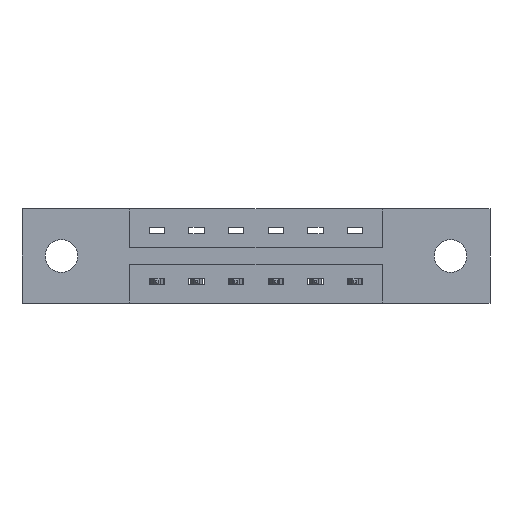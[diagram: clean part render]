
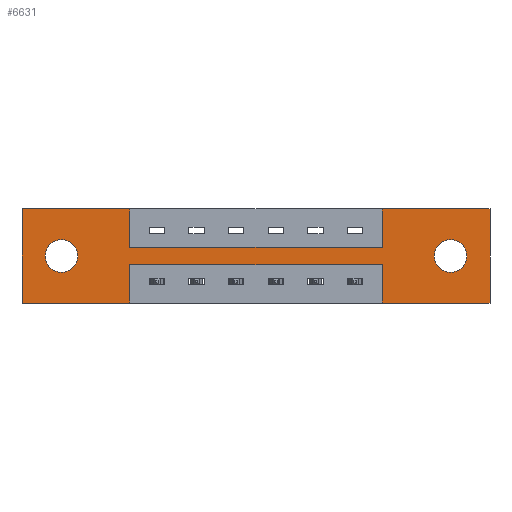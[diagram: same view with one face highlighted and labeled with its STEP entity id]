
A CAD part, front view. The second image highlights one B-rep face of the part: STEP entity #6631.
In plain terms, the highlighted planar face has unit normal (0, -1, 0).
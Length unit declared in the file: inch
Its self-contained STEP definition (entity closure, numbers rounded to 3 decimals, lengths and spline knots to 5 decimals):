
#16 = VERTEX_POINT ( 'NONE', #6132 ) ;
#101 = EDGE_LOOP ( 'NONE', ( #5256, #5325, #5389, #5403, #5441, #5453, #5477, #5502, #5543, #5580, #5597, #5687 ) ) ;
#127 = CIRCLE ( 'NONE', #4814, 0.064 ) ;
#151 = CARTESIAN_POINT ( 'NONE',  ( 1.417, 0., -0.15 ) ) ;
#160 = CARTESIAN_POINT ( 'NONE',  ( 0., 0., 0. ) ) ;
#182 = EDGE_CURVE ( 'NONE', #6004, #833, #659, .T. ) ;
#189 = CIRCLE ( 'NONE', #5176, 0.064 ) ;
#208 = DIRECTION ( 'NONE',  ( 0., 0., -1. ) ) ;
#209 = AXIS2_PLACEMENT_3D ( 'NONE', #7320, #3175, #2017 ) ;
#292 = CARTESIAN_POINT ( 'NONE',  ( 1.842, 0., -0.37 ) ) ;
#468 = DIRECTION ( 'NONE',  ( 1., 0., 0. ) ) ;
#531 = EDGE_CURVE ( 'NONE', #5519, #2962, #932, .T. ) ;
#544 = DIRECTION ( 'NONE',  ( -1., 0., 0. ) ) ;
#653 = CARTESIAN_POINT ( 'NONE',  ( 0.425, 0., 0. ) ) ;
#659 = LINE ( 'NONE', #3459, #2836 ) ;
#678 = VECTOR ( 'NONE', #828, 39.37008 ) ;
#758 = VECTOR ( 'NONE', #3365, 39.37008 ) ;
#828 = DIRECTION ( 'NONE',  ( -1., 0., 0. ) ) ;
#833 = VERTEX_POINT ( 'NONE', #1382 ) ;
#862 = EDGE_CURVE ( 'NONE', #2962, #3034, #5804, .T. ) ;
#932 = LINE ( 'NONE', #8737, #3050 ) ;
#995 = FACE_BOUND ( 'NONE', #5242, .T. ) ;
#1085 = EDGE_CURVE ( 'NONE', #6844, #3231, #1490, .T. ) ;
#1137 = DIRECTION ( 'NONE',  ( 0., 0., 1. ) ) ;
#1150 = CARTESIAN_POINT ( 'NONE',  ( 1.417, 0., 0. ) ) ;
#1175 = EDGE_CURVE ( 'NONE', #7182, #4051, #189, .T. ) ;
#1299 = EDGE_CURVE ( 'NONE', #16, #2086, #6705, .T. ) ;
#1382 = CARTESIAN_POINT ( 'NONE',  ( 0.425, 0., -0.15 ) ) ;
#1426 = VECTOR ( 'NONE', #468, 39.37008 ) ;
#1449 = CARTESIAN_POINT ( 'NONE',  ( 0.155, 0., -0.185 ) ) ;
#1450 = CARTESIAN_POINT ( 'NONE',  ( 0., 0., 0. ) ) ;
#1486 = EDGE_LOOP ( 'NONE', ( #5224, #5228 ) ) ;
#1490 = CIRCLE ( 'NONE', #1927, 0.064 ) ;
#1765 = EDGE_CURVE ( 'NONE', #3231, #6844, #127, .T. ) ;
#1921 = VECTOR ( 'NONE', #3232, 39.37008 ) ;
#1927 = AXIS2_PLACEMENT_3D ( 'NONE', #9051, #9048, #8872 ) ;
#1930 = DIRECTION ( 'NONE',  ( 0., 1., 0. ) ) ;
#1957 = EDGE_CURVE ( 'NONE', #4051, #7182, #5655, .T. ) ;
#1971 = EDGE_CURVE ( 'NONE', #8786, #16, #8321, .T. ) ;
#1974 = EDGE_CURVE ( 'NONE', #2156, #8786, #5214, .T. ) ;
#2004 = EDGE_CURVE ( 'NONE', #5467, #6004, #8154, .T. ) ;
#2017 = DIRECTION ( 'NONE',  ( 0., 0., 1. ) ) ;
#2056 = VECTOR ( 'NONE', #5476, 39.37008 ) ;
#2076 = DIRECTION ( 'NONE',  ( 0., 0., -1. ) ) ;
#2086 = VERTEX_POINT ( 'NONE', #8127 ) ;
#2118 = EDGE_CURVE ( 'NONE', #3034, #2156, #7721, .T. ) ;
#2144 = EDGE_CURVE ( 'NONE', #5333, #5519, #5849, .T. ) ;
#2156 = VERTEX_POINT ( 'NONE', #4858 ) ;
#2201 = CARTESIAN_POINT ( 'NONE',  ( 1.687, 0., -0.121 ) ) ;
#2596 = EDGE_CURVE ( 'NONE', #5442, #5333, #7430, .T. ) ;
#2836 = VECTOR ( 'NONE', #2979, 39.37008 ) ;
#2962 = VERTEX_POINT ( 'NONE', #292 ) ;
#2979 = DIRECTION ( 'NONE',  ( 0., 0., -1. ) ) ;
#3014 = DIRECTION ( 'NONE',  ( 0., 0., 1. ) ) ;
#3034 = VERTEX_POINT ( 'NONE', #6819 ) ;
#3050 = VECTOR ( 'NONE', #6617, 39.37008 ) ;
#3087 = DIRECTION ( 'NONE',  ( 0., 1., 0. ) ) ;
#3175 = DIRECTION ( 'NONE',  ( 0., 1., 0. ) ) ;
#3231 = VERTEX_POINT ( 'NONE', #2201 ) ;
#3232 = DIRECTION ( 'NONE',  ( 0., 0., 1. ) ) ;
#3365 = DIRECTION ( 'NONE',  ( 0., 0., 1. ) ) ;
#3459 = CARTESIAN_POINT ( 'NONE',  ( 0.425, 0., 0. ) ) ;
#3497 = CARTESIAN_POINT ( 'NONE',  ( 0., 0., 0. ) ) ;
#3514 = CARTESIAN_POINT ( 'NONE',  ( 0., 0., -0.37 ) ) ;
#3659 = AXIS2_PLACEMENT_3D ( 'NONE', #3514, #5097, #208 ) ;
#3684 = FACE_OUTER_BOUND ( 'NONE', #101, .T. ) ;
#3757 = VECTOR ( 'NONE', #1137, 39.37008 ) ;
#3913 = CARTESIAN_POINT ( 'NONE',  ( 0., 0., -0.37 ) ) ;
#4051 = VERTEX_POINT ( 'NONE', #6072 ) ;
#4287 = EDGE_CURVE ( 'NONE', #833, #5442, #7691, .T. ) ;
#4684 = EDGE_CURVE ( 'NONE', #2086, #5467, #6616, .T. ) ;
#4814 = AXIS2_PLACEMENT_3D ( 'NONE', #7879, #1930, #2076 ) ;
#4858 = CARTESIAN_POINT ( 'NONE',  ( 1.417, 0., -0.22 ) ) ;
#4985 = VECTOR ( 'NONE', #8726, 39.37008 ) ;
#5088 = DIRECTION ( 'NONE',  ( -1., 0., 0. ) ) ;
#5097 = DIRECTION ( 'NONE',  ( 0., -1., 0. ) ) ;
#5155 = VECTOR ( 'NONE', #544, 39.37008 ) ;
#5167 = ORIENTED_EDGE ( 'NONE', *, *, #1765, .T. ) ;
#5176 = AXIS2_PLACEMENT_3D ( 'NONE', #1449, #3087, #3014 ) ;
#5186 = CARTESIAN_POINT ( 'NONE',  ( 1.687, 0., -0.249 ) ) ;
#5214 = LINE ( 'NONE', #7357, #678 ) ;
#5216 = ORIENTED_EDGE ( 'NONE', *, *, #1085, .T. ) ;
#5224 = ORIENTED_EDGE ( 'NONE', *, *, #1957, .T. ) ;
#5228 = ORIENTED_EDGE ( 'NONE', *, *, #1175, .T. ) ;
#5242 = EDGE_LOOP ( 'NONE', ( #5167, #5216 ) ) ;
#5256 = ORIENTED_EDGE ( 'NONE', *, *, #1971, .F. ) ;
#5325 = ORIENTED_EDGE ( 'NONE', *, *, #1974, .F. ) ;
#5333 = VERTEX_POINT ( 'NONE', #6910 ) ;
#5389 = ORIENTED_EDGE ( 'NONE', *, *, #2118, .F. ) ;
#5403 = ORIENTED_EDGE ( 'NONE', *, *, #862, .F. ) ;
#5441 = ORIENTED_EDGE ( 'NONE', *, *, #531, .F. ) ;
#5442 = VERTEX_POINT ( 'NONE', #151 ) ;
#5453 = ORIENTED_EDGE ( 'NONE', *, *, #2144, .F. ) ;
#5467 = VERTEX_POINT ( 'NONE', #3497 ) ;
#5476 = DIRECTION ( 'NONE',  ( 1., 0., 0. ) ) ;
#5477 = ORIENTED_EDGE ( 'NONE', *, *, #2596, .F. ) ;
#5502 = ORIENTED_EDGE ( 'NONE', *, *, #4287, .F. ) ;
#5519 = VERTEX_POINT ( 'NONE', #7687 ) ;
#5543 = ORIENTED_EDGE ( 'NONE', *, *, #182, .F. ) ;
#5580 = ORIENTED_EDGE ( 'NONE', *, *, #2004, .F. ) ;
#5597 = ORIENTED_EDGE ( 'NONE', *, *, #4684, .F. ) ;
#5655 = CIRCLE ( 'NONE', #209, 0.064 ) ;
#5687 = ORIENTED_EDGE ( 'NONE', *, *, #1299, .F. ) ;
#5804 = LINE ( 'NONE', #3913, #6204 ) ;
#5849 = LINE ( 'NONE', #160, #1426 ) ;
#6004 = VERTEX_POINT ( 'NONE', #653 ) ;
#6013 = VECTOR ( 'NONE', #8285, 39.37008 ) ;
#6072 = CARTESIAN_POINT ( 'NONE',  ( 0.155, 0., -0.121 ) ) ;
#6132 = CARTESIAN_POINT ( 'NONE',  ( 0.425, 0., -0.37 ) ) ;
#6204 = VECTOR ( 'NONE', #5088, 39.37008 ) ;
#6616 = LINE ( 'NONE', #9091, #758 ) ;
#6617 = DIRECTION ( 'NONE',  ( 0., 0., -1. ) ) ;
#6631 = ADVANCED_FACE ( 'NONE', ( #995, #6792, #3684 ), #8226, .T. ) ;
#6648 = CARTESIAN_POINT ( 'NONE',  ( 0.425, 0., -0.37 ) ) ;
#6705 = LINE ( 'NONE', #8573, #5155 ) ;
#6792 = FACE_BOUND ( 'NONE', #1486, .T. ) ;
#6819 = CARTESIAN_POINT ( 'NONE',  ( 1.417, 0., -0.37 ) ) ;
#6844 = VERTEX_POINT ( 'NONE', #5186 ) ;
#6899 = CARTESIAN_POINT ( 'NONE',  ( 0.425, 0., -0.15 ) ) ;
#6910 = CARTESIAN_POINT ( 'NONE',  ( 1.417, 0., 0. ) ) ;
#7182 = VERTEX_POINT ( 'NONE', #7401 ) ;
#7320 = CARTESIAN_POINT ( 'NONE',  ( 0.155, 0., -0.185 ) ) ;
#7357 = CARTESIAN_POINT ( 'NONE',  ( 0.425, 0., -0.22 ) ) ;
#7401 = CARTESIAN_POINT ( 'NONE',  ( 0.155, 0., -0.249 ) ) ;
#7430 = LINE ( 'NONE', #1150, #3757 ) ;
#7687 = CARTESIAN_POINT ( 'NONE',  ( 1.842, 0., 0. ) ) ;
#7691 = LINE ( 'NONE', #6899, #6013 ) ;
#7721 = LINE ( 'NONE', #8427, #1921 ) ;
#7879 = CARTESIAN_POINT ( 'NONE',  ( 1.687, 0., -0.185 ) ) ;
#8127 = CARTESIAN_POINT ( 'NONE',  ( 0., 0., -0.37 ) ) ;
#8154 = LINE ( 'NONE', #1450, #2056 ) ;
#8226 = PLANE ( 'NONE',  #3659 ) ;
#8285 = DIRECTION ( 'NONE',  ( 1., 0., 0. ) ) ;
#8321 = LINE ( 'NONE', #6648, #4985 ) ;
#8427 = CARTESIAN_POINT ( 'NONE',  ( 1.417, 0., -0.37 ) ) ;
#8573 = CARTESIAN_POINT ( 'NONE',  ( 0., 0., -0.37 ) ) ;
#8726 = DIRECTION ( 'NONE',  ( 0., 0., -1. ) ) ;
#8737 = CARTESIAN_POINT ( 'NONE',  ( 1.842, 0., 0. ) ) ;
#8786 = VERTEX_POINT ( 'NONE', #8990 ) ;
#8872 = DIRECTION ( 'NONE',  ( 0., 0., -1. ) ) ;
#8990 = CARTESIAN_POINT ( 'NONE',  ( 0.425, 0., -0.22 ) ) ;
#9048 = DIRECTION ( 'NONE',  ( 0., 1., 0. ) ) ;
#9051 = CARTESIAN_POINT ( 'NONE',  ( 1.687, 0., -0.185 ) ) ;
#9091 = CARTESIAN_POINT ( 'NONE',  ( 0., 0., 0. ) ) ;
